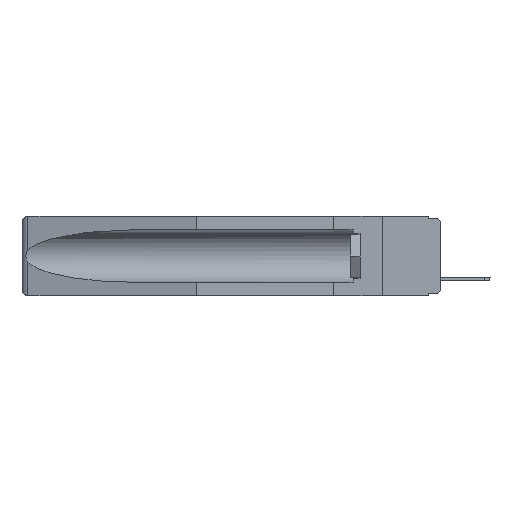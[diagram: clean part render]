
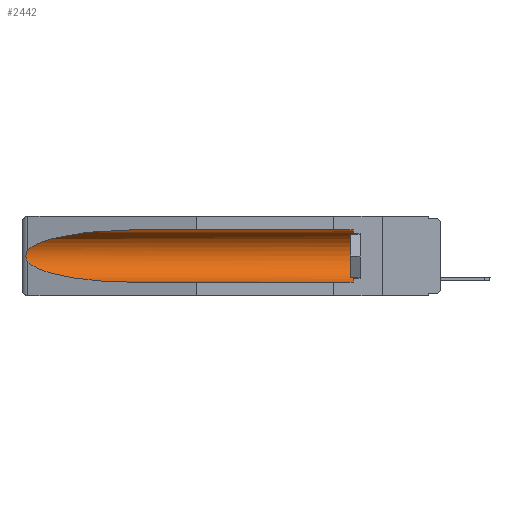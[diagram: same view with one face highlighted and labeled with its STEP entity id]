
A CAD part, left-side view. The second image highlights one B-rep face of the part: STEP entity #2442.
In plain terms, the highlighted cylindrical face has radius 2.857 mm (diameter 5.715 mm), a partial arc.
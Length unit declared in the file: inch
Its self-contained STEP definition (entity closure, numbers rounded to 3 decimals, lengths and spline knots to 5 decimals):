
#110 = CARTESIAN_POINT ( 'NONE',  ( 0.155, 0.126, -0.1715 ) ) ;
#411 = CARTESIAN_POINT ( 'NONE',  ( 0.155, 1.07973, -0.059 ) ) ;
#522 = CARTESIAN_POINT ( 'NONE',  ( 0.26655, 1.53094, -0.18657 ) ) ;
#613 = CARTESIAN_POINT ( 'NONE',  ( 0.26597, 1.5296, -0.19026 ) ) ;
#889 = AXIS2_PLACEMENT_3D ( 'NONE', #8589, #8789, #1096 ) ;
#1005 = LINE ( 'NONE', #16425, #12668 ) ;
#1096 = DIRECTION ( 'NONE',  ( 0., 0., 1. ) ) ;
#1644 = VERTEX_POINT ( 'NONE', #3985 ) ;
#1846 = EDGE_CURVE ( 'NONE', #4675, #5738, #19581, .T. ) ;
#2442 = ADVANCED_FACE ( 'NONE', ( #5359 ), #2610, .F. ) ;
#2610 = CYLINDRICAL_SURFACE ( 'NONE', #889, 0.1125 ) ;
#3072 = CARTESIAN_POINT ( 'NONE',  ( 0.155, 0.126, -0.284 ) ) ;
#3158 = CARTESIAN_POINT ( 'NONE',  ( 0.26537, 1.52718, -0.14972 ) ) ;
#3466 = CARTESIAN_POINT ( 'NONE',  ( 0.26654, 1.53092, -0.15636 ) ) ;
#3985 = CARTESIAN_POINT ( 'NONE',  ( 0.155, 1.07973, -0.059 ) ) ;
#4239 = DIRECTION ( 'NONE',  ( 0., 1., 0. ) ) ;
#4675 = VERTEX_POINT ( 'NONE', #3072 ) ;
#5359 = FACE_OUTER_BOUND ( 'NONE', #17973, .T. ) ;
#5419 = ORIENTED_EDGE ( 'NONE', *, *, #19886, .T. ) ;
#5738 = VERTEX_POINT ( 'NONE', #13543 ) ;
#6364 = ORIENTED_EDGE ( 'NONE', *, *, #10015, .T. ) ;
#6446 = EDGE_CURVE ( 'NONE', #14385, #6776, #7919, .T. ) ;
#6611 = EDGE_CURVE ( 'NONE', #5738, #1644, #1005, .T. ) ;
#6769 = ORIENTED_EDGE ( 'NONE', *, *, #14501, .F. ) ;
#6776 = VERTEX_POINT ( 'NONE', #7567 ) ;
#6864 = CARTESIAN_POINT ( 'NONE',  ( 0.26537, 1.52718, -0.14972 ) ) ;
#6901 = CARTESIAN_POINT ( 'NONE',  ( 0.26537, 1.52718, -0.14972 ) ) ;
#7567 = CARTESIAN_POINT ( 'NONE',  ( 0.26537, 1.52718, -0.19328 ) ) ;
#7607 = ORIENTED_EDGE ( 'NONE', *, *, #1846, .T. ) ;
#7868 =( BOUNDED_CURVE ( )  B_SPLINE_CURVE ( 3, ( #411, #11164, #11271, #3158 ),
 .UNSPECIFIED., .F., .F. ) 
 B_SPLINE_CURVE_WITH_KNOTS ( ( 4, 4 ),
 ( 4.71239, 6.08839 ),
 .UNSPECIFIED. ) 
 CURVE ( )  GEOMETRIC_REPRESENTATION_ITEM ( )  RATIONAL_B_SPLINE_CURVE ( ( 1., 0.848, 0.848, 1. ) ) 
 REPRESENTATION_ITEM ( '' )  );
#7919 = B_SPLINE_CURVE_WITH_KNOTS ( 'NONE', 3,
 ( #6864, #15927, #3466, #17375, #14590, #19005, #8095, #522, #613, #8203 ),
 .UNSPECIFIED., .F., .F.,
 ( 4, 2, 2, 2, 4 ),
 ( 0., 0.00029, 0.00058, 0.00087, 0.00117 ),
 .UNSPECIFIED. ) ;
#8095 = CARTESIAN_POINT ( 'NONE',  ( 0.2673, 1.53269, -0.17917 ) ) ;
#8203 = CARTESIAN_POINT ( 'NONE',  ( 0.26537, 1.52718, -0.19328 ) ) ;
#8526 = VERTEX_POINT ( 'NONE', #12861 ) ;
#8589 = CARTESIAN_POINT ( 'NONE',  ( 0.155, -0.30754, -0.1715 ) ) ;
#8789 = DIRECTION ( 'NONE',  ( 0., 1., 0. ) ) ;
#8848 = AXIS2_PLACEMENT_3D ( 'NONE', #110, #12299, #12503 ) ;
#10015 = EDGE_CURVE ( 'NONE', #6776, #8526, #13454, .T. ) ;
#11012 = CARTESIAN_POINT ( 'NONE',  ( 0.26537, 1.52718, -0.19328 ) ) ;
#11164 = CARTESIAN_POINT ( 'NONE',  ( 0.21114, 1.30732, -0.059 ) ) ;
#11271 = CARTESIAN_POINT ( 'NONE',  ( 0.25451, 1.48313, -0.09465 ) ) ;
#11984 = LINE ( 'NONE', #18601, #19969 ) ;
#12299 = DIRECTION ( 'NONE',  ( 0., -1., 0. ) ) ;
#12503 = DIRECTION ( 'NONE',  ( 0., 0., 1. ) ) ;
#12668 = VECTOR ( 'NONE', #4239, 39.37008 ) ;
#12861 = CARTESIAN_POINT ( 'NONE',  ( 0.155, 1.07973, -0.284 ) ) ;
#13454 =( BOUNDED_CURVE ( )  B_SPLINE_CURVE ( 3, ( #11012, #17111, #17013, #13946 ),
 .UNSPECIFIED., .F., .F. ) 
 B_SPLINE_CURVE_WITH_KNOTS ( ( 4, 4 ),
 ( 0.1948, 1.5708 ),
 .UNSPECIFIED. ) 
 CURVE ( )  GEOMETRIC_REPRESENTATION_ITEM ( )  RATIONAL_B_SPLINE_CURVE ( ( 1., 0.848, 0.848, 1. ) ) 
 REPRESENTATION_ITEM ( '' )  );
#13543 = CARTESIAN_POINT ( 'NONE',  ( 0.155, 0.126, -0.059 ) ) ;
#13946 = CARTESIAN_POINT ( 'NONE',  ( 0.155, 1.07973, -0.284 ) ) ;
#14032 = ORIENTED_EDGE ( 'NONE', *, *, #6611, .T. ) ;
#14385 = VERTEX_POINT ( 'NONE', #6901 ) ;
#14501 = EDGE_CURVE ( 'NONE', #4675, #8526, #11984, .T. ) ;
#14590 = CARTESIAN_POINT ( 'NONE',  ( 0.2675, 1.53308, -0.16763 ) ) ;
#15927 = CARTESIAN_POINT ( 'NONE',  ( 0.26597, 1.52961, -0.15275 ) ) ;
#16425 = CARTESIAN_POINT ( 'NONE',  ( 0.155, -0.30754, -0.059 ) ) ;
#16857 = DIRECTION ( 'NONE',  ( 0., 1., 0. ) ) ;
#17013 = CARTESIAN_POINT ( 'NONE',  ( 0.21114, 1.30732, -0.284 ) ) ;
#17111 = CARTESIAN_POINT ( 'NONE',  ( 0.25451, 1.48313, -0.24835 ) ) ;
#17375 = CARTESIAN_POINT ( 'NONE',  ( 0.2673, 1.5327, -0.16383 ) ) ;
#17973 = EDGE_LOOP ( 'NONE', ( #5419, #19747, #6364, #6769, #7607, #14032 ) ) ;
#18601 = CARTESIAN_POINT ( 'NONE',  ( 0.155, -0.30754, -0.284 ) ) ;
#19005 = CARTESIAN_POINT ( 'NONE',  ( 0.2675, 1.53308, -0.17534 ) ) ;
#19581 = CIRCLE ( 'NONE', #8848, 0.1125 ) ;
#19747 = ORIENTED_EDGE ( 'NONE', *, *, #6446, .T. ) ;
#19886 = EDGE_CURVE ( 'NONE', #1644, #14385, #7868, .T. ) ;
#19969 = VECTOR ( 'NONE', #16857, 39.37008 ) ;
